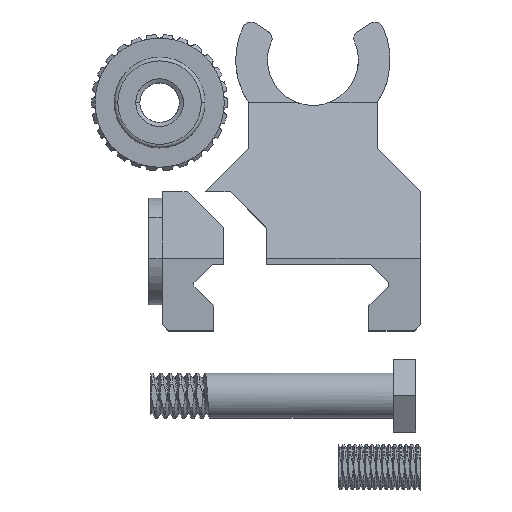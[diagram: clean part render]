
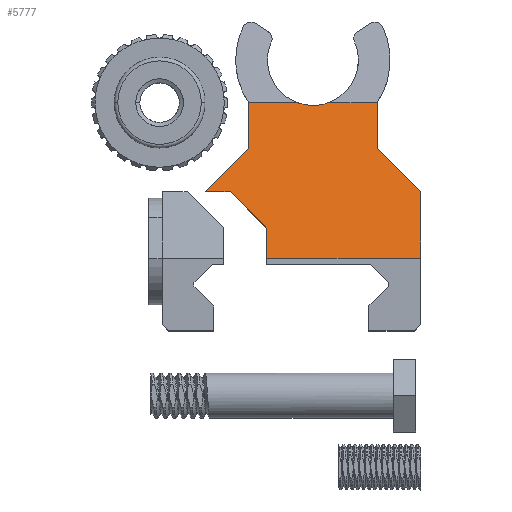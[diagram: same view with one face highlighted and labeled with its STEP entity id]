
A CAD part, top view. The second image highlights one B-rep face of the part: STEP entity #5777.
In plain terms, the highlighted planar face has unit normal (0, 0.281, 0.96).
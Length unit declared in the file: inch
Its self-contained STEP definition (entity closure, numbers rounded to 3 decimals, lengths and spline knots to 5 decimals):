
#431 = ORIENTED_EDGE ( 'NONE', *, *, #32367, .F. ) ;
#900 = CARTESIAN_POINT ( 'NONE',  ( -0.35347, 0.93168, 0.3697 ) ) ;
#2269 = CARTESIAN_POINT ( 'NONE',  ( -0.5925, 0.14418, 0.6 ) ) ;
#2695 = CARTESIAN_POINT ( 'NONE',  ( -0.6075, 0.495, 0.4974 ) ) ;
#3091 = CARTESIAN_POINT ( 'NONE',  ( -0.45525, 0.51, 0.49302 ) ) ;
#3230 = VECTOR ( 'NONE', #27131, 39.37008 ) ;
#3433 = CARTESIAN_POINT ( 'NONE',  ( 0.08257, 0.99903, 0.35 ) ) ;
#3664 = VERTEX_POINT ( 'NONE', #18942 ) ;
#3760 = EDGE_CURVE ( 'NONE', #31688, #24865, #24584, .T. ) ;
#4041 = LINE ( 'NONE', #6960, #3230 ) ;
#4290 = ORIENTED_EDGE ( 'NONE', *, *, #7850, .F. ) ;
#4412 = CARTESIAN_POINT ( 'NONE',  ( -0.5925, 0.99903, 0.35 ) ) ;
#4575 = LINE ( 'NONE', #12716, #27517 ) ;
#4932 = LINE ( 'NONE', #25453, #23333 ) ;
#5206 = DIRECTION ( 'NONE',  ( 0.692, 0.692, -0.203 ) ) ;
#5551 = ORIENTED_EDGE ( 'NONE', *, *, #25498, .F. ) ;
#5684 = FACE_OUTER_BOUND ( 'NONE', #10029, .T. ) ;
#5777 = ADVANCED_FACE ( 'NONE', ( #5684 ), #9407, .F. ) ;
#5852 = DIRECTION ( 'NONE',  ( -1., 0., 0. ) ) ;
#6261 = LINE ( 'NONE', #31951, #17663 ) ;
#6310 = VERTEX_POINT ( 'NONE', #14074 ) ;
#6960 = CARTESIAN_POINT ( 'NONE',  ( 0.35347, 0.93168, 0.3697 ) ) ;
#7652 = CARTESIAN_POINT ( 'NONE',  ( -0.08257, 0.99903, 0.35 ) ) ;
#7835 = ORIENTED_EDGE ( 'NONE', *, *, #16014, .F. ) ;
#7850 = EDGE_CURVE ( 'NONE', #24865, #28359, #30992, .T. ) ;
#8540 = CARTESIAN_POINT ( 'NONE',  ( -0.35347, 0.99903, 0.35 ) ) ;
#9083 = EDGE_CURVE ( 'NONE', #28359, #30245, #12524, .T. ) ;
#9192 = DIRECTION ( 'NONE',  ( 0., -0.281, -0.96 ) ) ;
#9231 = EDGE_CURVE ( 'NONE', #30797, #11339, #24448, .T. ) ;
#9407 = PLANE ( 'NONE',  #9707 ) ;
#9707 = AXIS2_PLACEMENT_3D ( 'NONE', #24821, #9192, #27474 ) ;
#9824 = VECTOR ( 'NONE', #21718, 39.37008 ) ;
#9969 = CARTESIAN_POINT ( 'NONE',  ( -0.02859, 0.98014, 0.35552 ) ) ;
#10029 = EDGE_LOOP ( 'NONE', ( #4290, #31234, #21562, #11575, #17865, #21154, #32414, #5551, #22430, #431, #7835, #14929 ) ) ;
#10830 = VERTEX_POINT ( 'NONE', #15835 ) ;
#11339 = VERTEX_POINT ( 'NONE', #13178 ) ;
#11575 = ORIENTED_EDGE ( 'NONE', *, *, #14517, .F. ) ;
#12524 =( BOUNDED_CURVE ( )  B_SPLINE_CURVE ( 3, ( #7652, #9969, #20666, #12701 ),
 .UNSPECIFIED., .F., .F. ) 
 B_SPLINE_CURVE_WITH_KNOTS ( ( 4, 4 ),
 ( 2.80501, 3.47818 ),
 .UNSPECIFIED. ) 
 CURVE ( )  GEOMETRIC_REPRESENTATION_ITEM ( )  RATIONAL_B_SPLINE_CURVE ( ( 1., 0.963, 0.963, 1. ) ) 
 REPRESENTATION_ITEM ( '' )  );
#12701 = CARTESIAN_POINT ( 'NONE',  ( 0.08257, 0.99903, 0.35 ) ) ;
#12702 = CARTESIAN_POINT ( 'NONE',  ( -0.25525, 0.31, 0.55151 ) ) ;
#12716 = CARTESIAN_POINT ( 'NONE',  ( 0.5925, -0.19282, 0.69856 ) ) ;
#13178 = CARTESIAN_POINT ( 'NONE',  ( 0.5925, 0.14418, 0.6 ) ) ;
#14074 = CARTESIAN_POINT ( 'NONE',  ( 0.35347, 0.74903, 0.42311 ) ) ;
#14208 = VECTOR ( 'NONE', #15412, 39.37008 ) ;
#14517 = EDGE_CURVE ( 'NONE', #23517, #3664, #28818, .T. ) ;
#14900 = VECTOR ( 'NONE', #5852, 39.37008 ) ;
#14929 = ORIENTED_EDGE ( 'NONE', *, *, #9083, .F. ) ;
#15412 = DIRECTION ( 'NONE',  ( 1., 0., 0. ) ) ;
#15461 = VECTOR ( 'NONE', #31392, 39.37008 ) ;
#15835 = CARTESIAN_POINT ( 'NONE',  ( 0.35347, 0.99903, 0.35 ) ) ;
#16014 = EDGE_CURVE ( 'NONE', #30245, #10830, #17306, .T. ) ;
#17306 = LINE ( 'NONE', #4412, #30047 ) ;
#17320 = CARTESIAN_POINT ( 'NONE',  ( -0.08257, 0.99903, 0.35 ) ) ;
#17663 = VECTOR ( 'NONE', #18752, 39.37008 ) ;
#17865 = ORIENTED_EDGE ( 'NONE', *, *, #20670, .T. ) ;
#17870 = CARTESIAN_POINT ( 'NONE',  ( -0.35347, 0.74903, 0.42311 ) ) ;
#18752 = DIRECTION ( 'NONE',  ( 0.692, -0.692, 0.203 ) ) ;
#18942 = CARTESIAN_POINT ( 'NONE',  ( -0.5925, 0.51, 0.49302 ) ) ;
#19138 = CARTESIAN_POINT ( 'NONE',  ( 0.5925, 0.51, 0.49302 ) ) ;
#19288 = VECTOR ( 'NONE', #5206, 39.37008 ) ;
#20666 = CARTESIAN_POINT ( 'NONE',  ( 0.02859, 0.98014, 0.35552 ) ) ;
#20670 = EDGE_CURVE ( 'NONE', #23517, #22447, #6261, .T. ) ;
#20765 = LINE ( 'NONE', #26222, #15461 ) ;
#21154 = ORIENTED_EDGE ( 'NONE', *, *, #27301, .F. ) ;
#21562 = ORIENTED_EDGE ( 'NONE', *, *, #27695, .F. ) ;
#21718 = DIRECTION ( 'NONE',  ( 0., 0.96, -0.281 ) ) ;
#22382 = DIRECTION ( 'NONE',  ( 1., 0., 0. ) ) ;
#22430 = ORIENTED_EDGE ( 'NONE', *, *, #31773, .F. ) ;
#22447 = VERTEX_POINT ( 'NONE', #12702 ) ;
#23333 = VECTOR ( 'NONE', #30646, 39.37008 ) ;
#23517 = VERTEX_POINT ( 'NONE', #3091 ) ;
#23826 = CARTESIAN_POINT ( 'NONE',  ( -0.5925, 0.99903, 0.35 ) ) ;
#24448 = LINE ( 'NONE', #2269, #14208 ) ;
#24584 = LINE ( 'NONE', #900, #9824 ) ;
#24821 = CARTESIAN_POINT ( 'NONE',  ( -0.5925, 0.99903, 0.35 ) ) ;
#24865 = VERTEX_POINT ( 'NONE', #8540 ) ;
#25370 = LINE ( 'NONE', #2695, #19288 ) ;
#25453 = CARTESIAN_POINT ( 'NONE',  ( -0.25525, 0.29694, 0.55533 ) ) ;
#25498 = EDGE_CURVE ( 'NONE', #31118, #11339, #4575, .T. ) ;
#26222 = CARTESIAN_POINT ( 'NONE',  ( 0.6075, 0.495, 0.4974 ) ) ;
#26815 = CARTESIAN_POINT ( 'NONE',  ( -0.25525, 0.14418, 0.6 ) ) ;
#26901 = CARTESIAN_POINT ( 'NONE',  ( 0.5925, 0.51, 0.49302 ) ) ;
#27131 = DIRECTION ( 'NONE',  ( 0., -0.96, 0.281 ) ) ;
#27301 = EDGE_CURVE ( 'NONE', #30797, #22447, #4932, .T. ) ;
#27474 = DIRECTION ( 'NONE',  ( 0., 0.96, -0.281 ) ) ;
#27517 = VECTOR ( 'NONE', #28500, 39.37008 ) ;
#27695 = EDGE_CURVE ( 'NONE', #3664, #31688, #25370, .T. ) ;
#28359 = VERTEX_POINT ( 'NONE', #17320 ) ;
#28500 = DIRECTION ( 'NONE',  ( 0., -0.96, 0.281 ) ) ;
#28818 = LINE ( 'NONE', #26901, #14900 ) ;
#30047 = VECTOR ( 'NONE', #22382, 39.37008 ) ;
#30245 = VERTEX_POINT ( 'NONE', #3433 ) ;
#30619 = VECTOR ( 'NONE', #31503, 39.37008 ) ;
#30646 = DIRECTION ( 'NONE',  ( 0., 0.96, -0.281 ) ) ;
#30797 = VERTEX_POINT ( 'NONE', #26815 ) ;
#30992 = LINE ( 'NONE', #23826, #30619 ) ;
#31118 = VERTEX_POINT ( 'NONE', #19138 ) ;
#31234 = ORIENTED_EDGE ( 'NONE', *, *, #3760, .F. ) ;
#31392 = DIRECTION ( 'NONE',  ( 0.692, -0.692, 0.203 ) ) ;
#31503 = DIRECTION ( 'NONE',  ( 1., 0., 0. ) ) ;
#31688 = VERTEX_POINT ( 'NONE', #17870 ) ;
#31773 = EDGE_CURVE ( 'NONE', #6310, #31118, #20765, .T. ) ;
#31951 = CARTESIAN_POINT ( 'NONE',  ( -0.36218, 0.41693, 0.52023 ) ) ;
#32367 = EDGE_CURVE ( 'NONE', #10830, #6310, #4041, .T. ) ;
#32414 = ORIENTED_EDGE ( 'NONE', *, *, #9231, .T. ) ;
